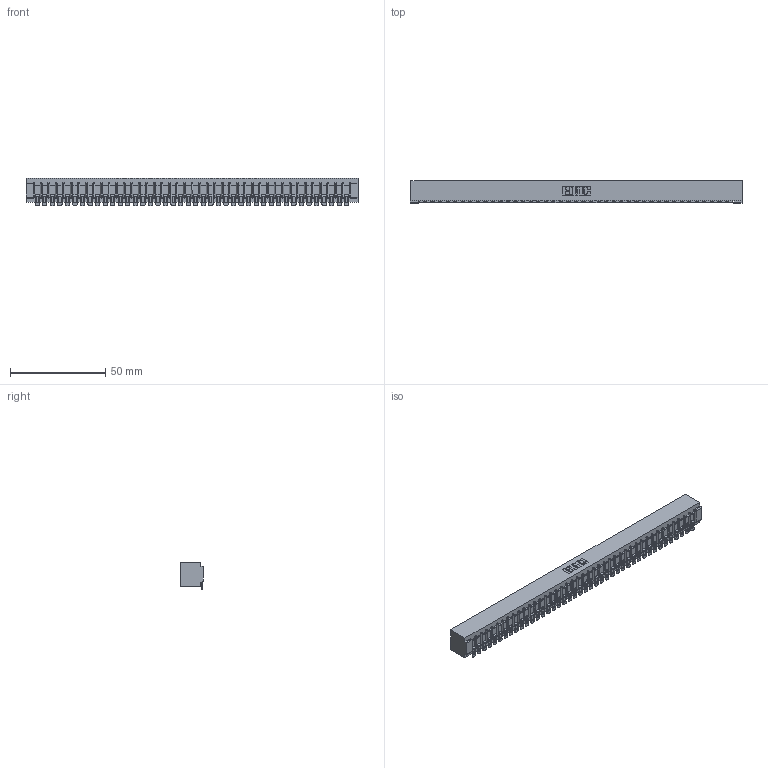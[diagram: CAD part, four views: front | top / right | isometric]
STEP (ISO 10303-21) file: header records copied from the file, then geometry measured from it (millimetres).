
FILE_DESCRIPTION (( 'STEP AP203' ), '1' );
FILE_NAME ('307-042-454-101.STEP', '2020-09-29T18:16:16', ( '' ), ( '' ), 'SwSTEP 2.0', 'SolidWorks 2020', '' );
FILE_SCHEMA (( 'CONFIG_CONTROL_DESIGN' ));
Length unit declared in the file: inch
Products named in the file (3): 307-042-454-101; 307-290-002_554; 307 Part_No Mounting Lugs
Assembly tree (43 placements, depth 2):
  307-042-454-101
    307 Part_No Mounting Lugs
    307-290-002_554  x42
Bounding box: 174.29 x 12.01 x 14.52 mm (x, y, z)
Volume: 19224.6 mm3; surface area: 24683.5 mm2
Topology: 43 solids, 43 shells, 3555 faces, 10925 edges, 7166 vertices
Faces by surface type: plane 1998, cylinder 1471, sphere 86
Entity records: 36693 total; most frequent: CARTESIAN_POINT 6190, ORIENTED_EDGE 6180, DIRECTION 6018, EDGE_CURVE 3090, VECTOR 2362, LINE 2362, VERTEX_POINT 2000, AXIS2_PLACEMENT_3D 1828
